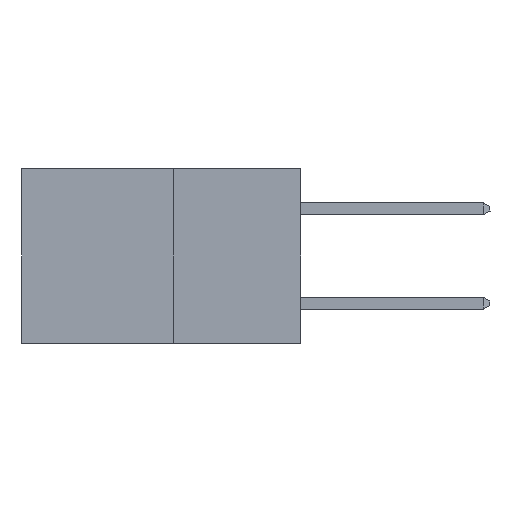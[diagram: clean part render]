
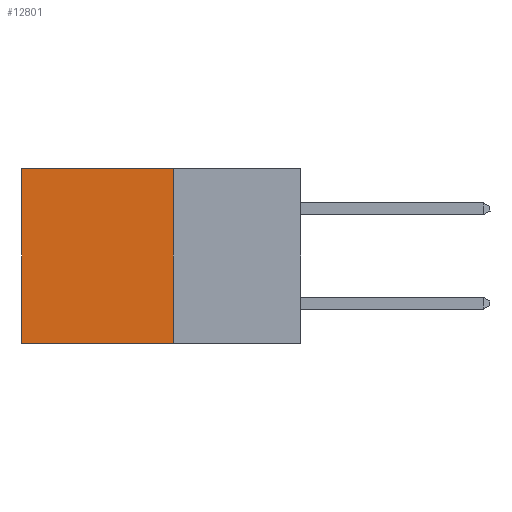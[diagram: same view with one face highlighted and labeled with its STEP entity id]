
A CAD part, left-side view. The second image highlights one B-rep face of the part: STEP entity #12801.
In plain terms, the highlighted planar face has unit normal (-1, 0, 0).
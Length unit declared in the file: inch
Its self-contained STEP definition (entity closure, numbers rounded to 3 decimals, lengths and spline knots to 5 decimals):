
#1292 = LINE ( 'NONE', #2159, #5010 ) ;
#1668 = DIRECTION ( 'NONE',  ( 0., 0., -1. ) ) ;
#1956 = CARTESIAN_POINT ( 'NONE',  ( 0.277, 0.27, -0.37 ) ) ;
#2159 = CARTESIAN_POINT ( 'NONE',  ( 0.277, 0.27, -0.37 ) ) ;
#2613 = ORIENTED_EDGE ( 'NONE', *, *, #13080, .T. ) ;
#3137 = EDGE_CURVE ( 'NONE', #3544, #15415, #18694, .T. ) ;
#3544 = VERTEX_POINT ( 'NONE', #18679 ) ;
#3837 = DIRECTION ( 'NONE',  ( 0., 0., -1. ) ) ;
#4919 = DIRECTION ( 'NONE',  ( 0., 1., 0. ) ) ;
#5010 = VECTOR ( 'NONE', #3837, 39.37008 ) ;
#5317 = DIRECTION ( 'NONE',  ( 0., 1., 0. ) ) ;
#5447 = EDGE_CURVE ( 'NONE', #18350, #15415, #14142, .T. ) ;
#5858 = CARTESIAN_POINT ( 'NONE',  ( 0.277, 0.27, -0.37 ) ) ;
#6189 = VECTOR ( 'NONE', #4919, 39.37008 ) ;
#6903 = VERTEX_POINT ( 'NONE', #12204 ) ;
#7644 = LINE ( 'NONE', #15698, #18779 ) ;
#7908 = FACE_OUTER_BOUND ( 'NONE', #18844, .T. ) ;
#7913 = PLANE ( 'NONE',  #16386 ) ;
#8857 = ORIENTED_EDGE ( 'NONE', *, *, #11231, .F. ) ;
#8871 = CARTESIAN_POINT ( 'NONE',  ( 0.277, 0.59, -0.37 ) ) ;
#9268 = ORIENTED_EDGE ( 'NONE', *, *, #3137, .T. ) ;
#9500 = CARTESIAN_POINT ( 'NONE',  ( 0.277, 0.27, -0.37 ) ) ;
#10758 = DIRECTION ( 'NONE',  ( 0., 0., -1. ) ) ;
#10976 = CARTESIAN_POINT ( 'NONE',  ( 0.277, 0.59, -0.37 ) ) ;
#10997 = DIRECTION ( 'NONE',  ( 1., 0., 0. ) ) ;
#11231 = EDGE_CURVE ( 'NONE', #6903, #18350, #1292, .T. ) ;
#11587 = ORIENTED_EDGE ( 'NONE', *, *, #5447, .F. ) ;
#12204 = CARTESIAN_POINT ( 'NONE',  ( 0.277, 0.27, 0. ) ) ;
#12801 = ADVANCED_FACE ( 'NONE', ( #7908 ), #7913, .F. ) ;
#13080 = EDGE_CURVE ( 'NONE', #6903, #3544, #7644, .T. ) ;
#14142 = LINE ( 'NONE', #1956, #6189 ) ;
#14503 = VECTOR ( 'NONE', #10758, 39.37008 ) ;
#15415 = VERTEX_POINT ( 'NONE', #8871 ) ;
#15698 = CARTESIAN_POINT ( 'NONE',  ( 0.277, 0.27, 0. ) ) ;
#16386 = AXIS2_PLACEMENT_3D ( 'NONE', #9500, #10997, #1668 ) ;
#18350 = VERTEX_POINT ( 'NONE', #5858 ) ;
#18679 = CARTESIAN_POINT ( 'NONE',  ( 0.277, 0.59, 0. ) ) ;
#18694 = LINE ( 'NONE', #10976, #14503 ) ;
#18779 = VECTOR ( 'NONE', #5317, 39.37008 ) ;
#18844 = EDGE_LOOP ( 'NONE', ( #9268, #11587, #8857, #2613 ) ) ;
